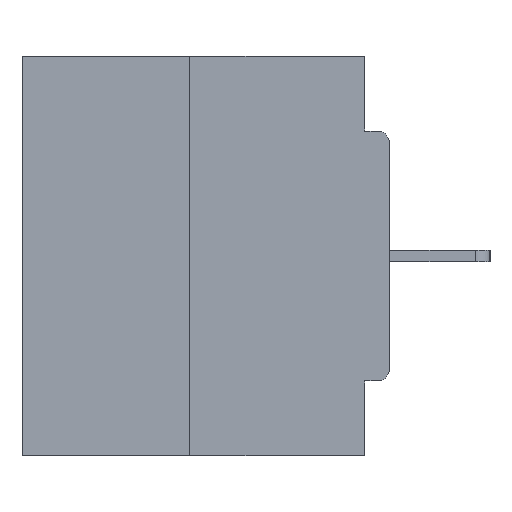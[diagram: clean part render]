
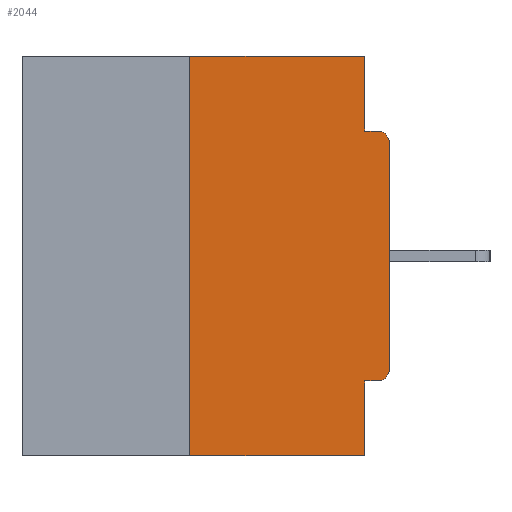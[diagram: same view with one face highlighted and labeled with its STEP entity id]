
A CAD part, left-side view. The second image highlights one B-rep face of the part: STEP entity #2044.
In plain terms, the highlighted planar face has unit normal (-1, 0, 0).
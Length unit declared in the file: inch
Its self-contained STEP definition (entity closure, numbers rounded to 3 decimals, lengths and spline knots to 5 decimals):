
#601 = CIRCLE ( 'NONE', #5002, 0.015 ) ;
#605 = CARTESIAN_POINT ( 'NONE',  ( 0., 0.031, -0.4065 ) ) ;
#1006 = EDGE_CURVE ( 'NONE', #2438, #2683, #22074, .T. ) ;
#1255 = CARTESIAN_POINT ( 'NONE',  ( 0., 0.031, -0.5 ) ) ;
#1474 = LINE ( 'NONE', #32876, #15518 ) ;
#1598 = AXIS2_PLACEMENT_3D ( 'NONE', #12806, #22903, #25820 ) ;
#2044 = ADVANCED_FACE ( 'NONE', ( #10569 ), #12625, .F. ) ;
#2438 = VERTEX_POINT ( 'NONE', #32507 ) ;
#2683 = VERTEX_POINT ( 'NONE', #8123 ) ;
#3594 = EDGE_CURVE ( 'NONE', #33320, #7022, #27006, .T. ) ;
#3666 = ORIENTED_EDGE ( 'NONE', *, *, #3594, .F. ) ;
#3885 = VECTOR ( 'NONE', #29413, 39.37008 ) ;
#3919 = VERTEX_POINT ( 'NONE', #12592 ) ;
#4835 = EDGE_CURVE ( 'NONE', #23375, #16516, #21071, .T. ) ;
#4855 = CARTESIAN_POINT ( 'NONE',  ( 0., 0.031, -0.0935 ) ) ;
#4897 = DIRECTION ( 'NONE',  ( -1., 0., 0. ) ) ;
#5002 = AXIS2_PLACEMENT_3D ( 'NONE', #12383, #30910, #28316 ) ;
#5359 = LINE ( 'NONE', #31258, #31123 ) ;
#6362 = LINE ( 'NONE', #18870, #9059 ) ;
#6660 = LINE ( 'NONE', #9217, #32744 ) ;
#7022 = VERTEX_POINT ( 'NONE', #4855 ) ;
#7304 = AXIS2_PLACEMENT_3D ( 'NONE', #21170, #4897, #23256 ) ;
#7750 = EDGE_CURVE ( 'NONE', #20052, #16516, #6660, .T. ) ;
#7761 = EDGE_CURVE ( 'NONE', #23375, #10217, #29801, .T. ) ;
#7891 = CARTESIAN_POINT ( 'NONE',  ( 0., 0., -0.4065 ) ) ;
#8056 = DIRECTION ( 'NONE',  ( 0., -1., 0. ) ) ;
#8123 = CARTESIAN_POINT ( 'NONE',  ( 0., 0., -0.3915 ) ) ;
#8343 = CARTESIAN_POINT ( 'NONE',  ( 0., 0.031, 0. ) ) ;
#8726 = ORIENTED_EDGE ( 'NONE', *, *, #4835, .T. ) ;
#9059 = VECTOR ( 'NONE', #16792, 39.37008 ) ;
#9217 = CARTESIAN_POINT ( 'NONE',  ( 0., 0.031, -0.5 ) ) ;
#9383 = DIRECTION ( 'NONE',  ( 0., 0., 1. ) ) ;
#9733 = ORIENTED_EDGE ( 'NONE', *, *, #7761, .F. ) ;
#10202 = VECTOR ( 'NONE', #28789, 39.37008 ) ;
#10217 = VERTEX_POINT ( 'NONE', #30382 ) ;
#10569 = FACE_OUTER_BOUND ( 'NONE', #22961, .T. ) ;
#11540 = CARTESIAN_POINT ( 'NONE',  ( 0., 0.25, -0.5 ) ) ;
#11918 = VECTOR ( 'NONE', #22250, 39.37008 ) ;
#12383 = CARTESIAN_POINT ( 'NONE',  ( 0., 0.015, -0.1085 ) ) ;
#12592 = CARTESIAN_POINT ( 'NONE',  ( 0., 0., -0.1085 ) ) ;
#12625 = PLANE ( 'NONE',  #1598 ) ;
#12806 = CARTESIAN_POINT ( 'NONE',  ( 0., 0.46, 0. ) ) ;
#13266 = EDGE_CURVE ( 'NONE', #2438, #20052, #21574, .T. ) ;
#13727 = ORIENTED_EDGE ( 'NONE', *, *, #27782, .T. ) ;
#15460 = ORIENTED_EDGE ( 'NONE', *, *, #17963, .F. ) ;
#15518 = VECTOR ( 'NONE', #9383, 39.37008 ) ;
#16516 = VERTEX_POINT ( 'NONE', #1255 ) ;
#16788 = EDGE_CURVE ( 'NONE', #10217, #33320, #5359, .T. ) ;
#16792 = DIRECTION ( 'NONE',  ( 0., -1., 0. ) ) ;
#17963 = EDGE_CURVE ( 'NONE', #7022, #31242, #6362, .T. ) ;
#18870 = CARTESIAN_POINT ( 'NONE',  ( 0., 0., -0.0935 ) ) ;
#19047 = ORIENTED_EDGE ( 'NONE', *, *, #13266, .F. ) ;
#19107 = CARTESIAN_POINT ( 'NONE',  ( 0., 0.031, 0. ) ) ;
#19161 = VECTOR ( 'NONE', #8056, 39.37008 ) ;
#20052 = VERTEX_POINT ( 'NONE', #605 ) ;
#21071 = LINE ( 'NONE', #31541, #19161 ) ;
#21170 = CARTESIAN_POINT ( 'NONE',  ( 0., 0.015, -0.3915 ) ) ;
#21574 = LINE ( 'NONE', #7891, #10202 ) ;
#22074 = CIRCLE ( 'NONE', #7304, 0.015 ) ;
#22250 = DIRECTION ( 'NONE',  ( 0., 0., 1. ) ) ;
#22903 = DIRECTION ( 'NONE',  ( 1., 0., 0. ) ) ;
#22961 = EDGE_LOOP ( 'NONE', ( #30616, #9733, #8726, #31298, #19047, #30036, #27098, #13727, #15460, #3666 ) ) ;
#23256 = DIRECTION ( 'NONE',  ( 0., 0., -1. ) ) ;
#23375 = VERTEX_POINT ( 'NONE', #11540 ) ;
#24803 = CARTESIAN_POINT ( 'NONE',  ( 0., 0.25, 0. ) ) ;
#25820 = DIRECTION ( 'NONE',  ( 0., 0., -1. ) ) ;
#27006 = LINE ( 'NONE', #8343, #3885 ) ;
#27098 = ORIENTED_EDGE ( 'NONE', *, *, #31763, .T. ) ;
#27782 = EDGE_CURVE ( 'NONE', #3919, #31242, #601, .T. ) ;
#28316 = DIRECTION ( 'NONE',  ( 0., 0., -1. ) ) ;
#28789 = DIRECTION ( 'NONE',  ( 0., 1., 0. ) ) ;
#29413 = DIRECTION ( 'NONE',  ( 0., 0., -1. ) ) ;
#29664 = CARTESIAN_POINT ( 'NONE',  ( 0., 0.015, -0.0935 ) ) ;
#29801 = LINE ( 'NONE', #24803, #11918 ) ;
#30036 = ORIENTED_EDGE ( 'NONE', *, *, #1006, .T. ) ;
#30382 = CARTESIAN_POINT ( 'NONE',  ( 0., 0.25, 0. ) ) ;
#30616 = ORIENTED_EDGE ( 'NONE', *, *, #16788, .F. ) ;
#30910 = DIRECTION ( 'NONE',  ( -1., 0., 0. ) ) ;
#31089 = DIRECTION ( 'NONE',  ( 0., -1., 0. ) ) ;
#31123 = VECTOR ( 'NONE', #31089, 39.37008 ) ;
#31242 = VERTEX_POINT ( 'NONE', #29664 ) ;
#31258 = CARTESIAN_POINT ( 'NONE',  ( 0., 0.46, 0. ) ) ;
#31298 = ORIENTED_EDGE ( 'NONE', *, *, #7750, .F. ) ;
#31541 = CARTESIAN_POINT ( 'NONE',  ( 0., 0.46, -0.5 ) ) ;
#31763 = EDGE_CURVE ( 'NONE', #2683, #3919, #1474, .T. ) ;
#32507 = CARTESIAN_POINT ( 'NONE',  ( 0., 0.015, -0.4065 ) ) ;
#32551 = DIRECTION ( 'NONE',  ( 0., 0., -1. ) ) ;
#32744 = VECTOR ( 'NONE', #32551, 39.37008 ) ;
#32876 = CARTESIAN_POINT ( 'NONE',  ( 0., 0., 0. ) ) ;
#33320 = VERTEX_POINT ( 'NONE', #19107 ) ;
